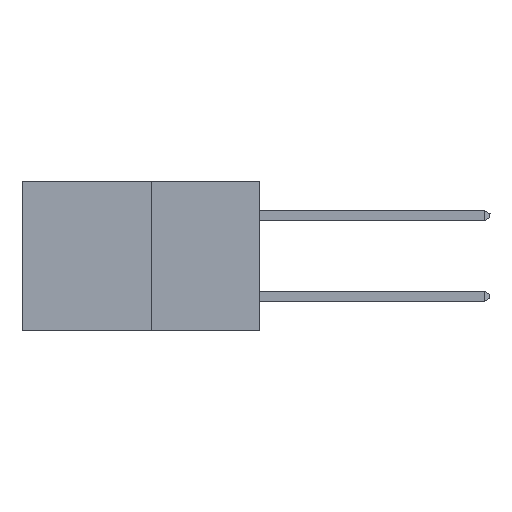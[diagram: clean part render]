
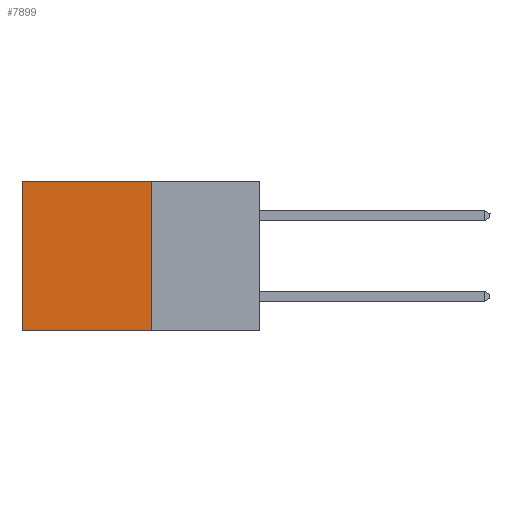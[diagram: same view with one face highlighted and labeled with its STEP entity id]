
A CAD part, left-side view. The second image highlights one B-rep face of the part: STEP entity #7899.
In plain terms, the highlighted planar face has unit normal (-1, 0, 0).
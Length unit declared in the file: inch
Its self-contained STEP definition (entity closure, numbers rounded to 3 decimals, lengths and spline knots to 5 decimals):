
#277 = ORIENTED_EDGE ( 'NONE', *, *, #4219, .T. ) ;
#374 = CARTESIAN_POINT ( 'NONE',  ( 0.277, 0.27, 0. ) ) ;
#391 = ORIENTED_EDGE ( 'NONE', *, *, #3114, .F. ) ;
#436 = AXIS2_PLACEMENT_3D ( 'NONE', #549, #513, #467 ) ;
#454 = VERTEX_POINT ( 'NONE', #809 ) ;
#467 = DIRECTION ( 'NONE',  ( 0., 0., -1. ) ) ;
#513 = DIRECTION ( 'NONE',  ( 1., 0., 0. ) ) ;
#546 = LINE ( 'NONE', #5510, #6366 ) ;
#549 = CARTESIAN_POINT ( 'NONE',  ( 0.277, 0.27, -0.37 ) ) ;
#564 = CARTESIAN_POINT ( 'NONE',  ( 0.277, 0.27, -0.37 ) ) ;
#614 = PLANE ( 'NONE',  #436 ) ;
#779 = VECTOR ( 'NONE', #7693, 39.37008 ) ;
#809 = CARTESIAN_POINT ( 'NONE',  ( 0.277, 0.27, -0.37 ) ) ;
#830 = DIRECTION ( 'NONE',  ( 0., 0., -1. ) ) ;
#1013 = LINE ( 'NONE', #564, #779 ) ;
#1016 = DIRECTION ( 'NONE',  ( 0., 1., 0. ) ) ;
#1073 = VECTOR ( 'NONE', #1016, 39.37008 ) ;
#1826 = CARTESIAN_POINT ( 'NONE',  ( 0.277, 0.59, 0. ) ) ;
#1905 = VERTEX_POINT ( 'NONE', #1826 ) ;
#1987 = CARTESIAN_POINT ( 'NONE',  ( 0.277, 0.27, 0. ) ) ;
#2921 = ORIENTED_EDGE ( 'NONE', *, *, #8374, .F. ) ;
#3114 = EDGE_CURVE ( 'NONE', #7628, #454, #1013, .T. ) ;
#3333 = VERTEX_POINT ( 'NONE', #4028 ) ;
#4028 = CARTESIAN_POINT ( 'NONE',  ( 0.277, 0.59, -0.37 ) ) ;
#4219 = EDGE_CURVE ( 'NONE', #1905, #3333, #546, .T. ) ;
#5293 = LINE ( 'NONE', #374, #5514 ) ;
#5486 = DIRECTION ( 'NONE',  ( 0., 1., 0. ) ) ;
#5510 = CARTESIAN_POINT ( 'NONE',  ( 0.277, 0.59, -0.37 ) ) ;
#5514 = VECTOR ( 'NONE', #5486, 39.37008 ) ;
#6366 = VECTOR ( 'NONE', #830, 39.37008 ) ;
#6629 = FACE_OUTER_BOUND ( 'NONE', #8539, .T. ) ;
#6799 = CARTESIAN_POINT ( 'NONE',  ( 0.277, 0.27, -0.37 ) ) ;
#7400 = ORIENTED_EDGE ( 'NONE', *, *, #8861, .T. ) ;
#7628 = VERTEX_POINT ( 'NONE', #1987 ) ;
#7693 = DIRECTION ( 'NONE',  ( 0., 0., -1. ) ) ;
#7899 = ADVANCED_FACE ( 'NONE', ( #6629 ), #614, .F. ) ;
#8374 = EDGE_CURVE ( 'NONE', #454, #3333, #8448, .T. ) ;
#8448 = LINE ( 'NONE', #6799, #1073 ) ;
#8539 = EDGE_LOOP ( 'NONE', ( #277, #2921, #391, #7400 ) ) ;
#8861 = EDGE_CURVE ( 'NONE', #7628, #1905, #5293, .T. ) ;
